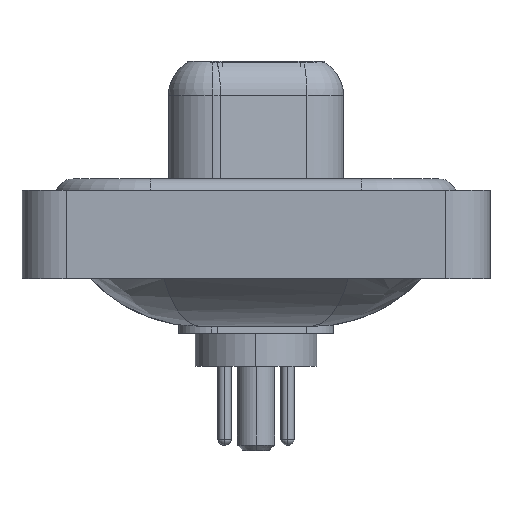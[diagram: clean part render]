
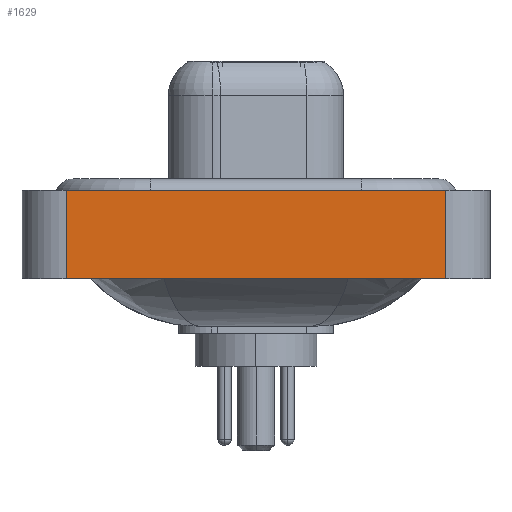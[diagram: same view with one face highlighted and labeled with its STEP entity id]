
A CAD part, left-side view. The second image highlights one B-rep face of the part: STEP entity #1629.
In plain terms, the highlighted planar face has unit normal (-1, 0, 0).
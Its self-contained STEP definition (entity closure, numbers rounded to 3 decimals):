
#1380 = DIRECTION ( 'NONE',  ( 0., 0., 1. ) ) ;
#1629 = ADVANCED_FACE ( 'NONE', ( #12782 ), #16608, .T. ) ;
#1889 = CARTESIAN_POINT ( 'NONE',  ( -7.35, -8.55, -3.6 ) ) ;
#3563 = ORIENTED_EDGE ( 'NONE', *, *, #20423, .T. ) ;
#3873 = VECTOR ( 'NONE', #15423, 1000. ) ;
#5719 = EDGE_CURVE ( 'NONE', #22749, #22693, #17607, .T. ) ;
#6920 = EDGE_CURVE ( 'NONE', #14569, #22693, #22899, .T. ) ;
#7252 = DIRECTION ( 'NONE',  ( 0., 0., 1. ) ) ;
#7360 = VECTOR ( 'NONE', #19097, 1000. ) ;
#7425 = DIRECTION ( 'NONE',  ( 0., -1., 0. ) ) ;
#7622 = VERTEX_POINT ( 'NONE', #12650 ) ;
#7995 = CARTESIAN_POINT ( 'NONE',  ( -7.35, -8.55, 0.4 ) ) ;
#8778 = CARTESIAN_POINT ( 'NONE',  ( -7.35, -8.55, -3.6 ) ) ;
#10251 = DIRECTION ( 'NONE',  ( -1., 0., 0. ) ) ;
#10672 = EDGE_CURVE ( 'NONE', #7622, #22749, #10849, .T. ) ;
#10734 = CARTESIAN_POINT ( 'NONE',  ( -7.35, 8.55, 0.4 ) ) ;
#10849 = LINE ( 'NONE', #24105, #16706 ) ;
#11833 = VECTOR ( 'NONE', #7425, 1000. ) ;
#12650 = CARTESIAN_POINT ( 'NONE',  ( -7.35, 8.55, -3.6 ) ) ;
#12782 = FACE_OUTER_BOUND ( 'NONE', #20982, .T. ) ;
#13636 = CARTESIAN_POINT ( 'NONE',  ( -7.35, -8.55, -3.6 ) ) ;
#14569 = VERTEX_POINT ( 'NONE', #13636 ) ;
#15423 = DIRECTION ( 'NONE',  ( 0., -1., 0. ) ) ;
#15654 = AXIS2_PLACEMENT_3D ( 'NONE', #23384, #10251, #7252 ) ;
#15754 = ORIENTED_EDGE ( 'NONE', *, *, #5719, .F. ) ;
#16608 = PLANE ( 'NONE',  #15654 ) ;
#16706 = VECTOR ( 'NONE', #1380, 1000. ) ;
#17607 = LINE ( 'NONE', #7995, #3873 ) ;
#19097 = DIRECTION ( 'NONE',  ( 0., 0., 1. ) ) ;
#19472 = CARTESIAN_POINT ( 'NONE',  ( -7.35, -8.55, 0.4 ) ) ;
#19706 = ORIENTED_EDGE ( 'NONE', *, *, #6920, .T. ) ;
#20423 = EDGE_CURVE ( 'NONE', #7622, #14569, #24016, .T. ) ;
#20982 = EDGE_LOOP ( 'NONE', ( #19706, #15754, #21274, #3563 ) ) ;
#21274 = ORIENTED_EDGE ( 'NONE', *, *, #10672, .F. ) ;
#22693 = VERTEX_POINT ( 'NONE', #19472 ) ;
#22749 = VERTEX_POINT ( 'NONE', #10734 ) ;
#22899 = LINE ( 'NONE', #1889, #7360 ) ;
#23384 = CARTESIAN_POINT ( 'NONE',  ( -7.35, -8.55, -3.6 ) ) ;
#24016 = LINE ( 'NONE', #8778, #11833 ) ;
#24105 = CARTESIAN_POINT ( 'NONE',  ( -7.35, 8.55, -3.6 ) ) ;
